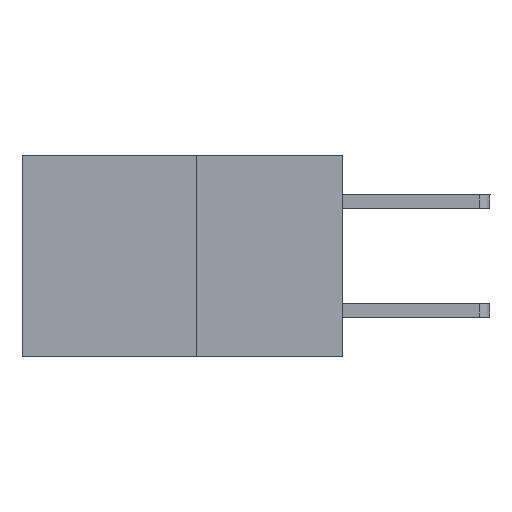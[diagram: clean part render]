
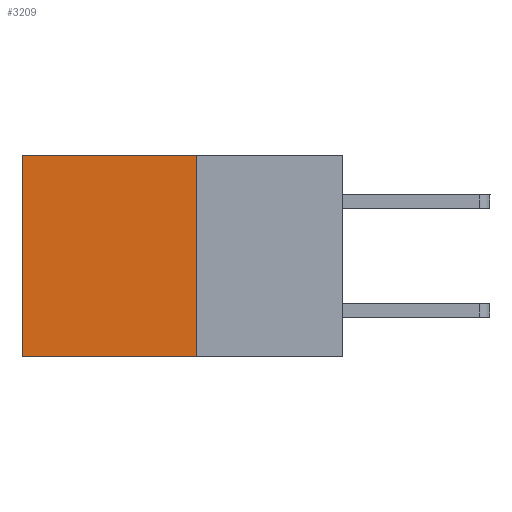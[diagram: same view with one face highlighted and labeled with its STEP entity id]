
A CAD part, left-side view. The second image highlights one B-rep face of the part: STEP entity #3209.
In plain terms, the highlighted planar face has unit normal (-1, 0, 0).
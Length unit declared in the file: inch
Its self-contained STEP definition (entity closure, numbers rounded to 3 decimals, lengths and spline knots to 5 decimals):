
#361 = VERTEX_POINT ( 'NONE', #5251 ) ;
#444 = CARTESIAN_POINT ( 'NONE',  ( 0.277, 0.27, -0.37 ) ) ;
#500 = DIRECTION ( 'NONE',  ( 0., 1., 0. ) ) ;
#676 = CARTESIAN_POINT ( 'NONE',  ( 0.277, 0.59, 0. ) ) ;
#831 = VERTEX_POINT ( 'NONE', #676 ) ;
#997 = VECTOR ( 'NONE', #500, 39.37008 ) ;
#1170 = ORIENTED_EDGE ( 'NONE', *, *, #3942, .F. ) ;
#1410 = LINE ( 'NONE', #3050, #6306 ) ;
#1750 = EDGE_CURVE ( 'NONE', #9320, #831, #1410, .T. ) ;
#1763 = LINE ( 'NONE', #9527, #6383 ) ;
#2321 = DIRECTION ( 'NONE',  ( 0., 0., -1. ) ) ;
#3050 = CARTESIAN_POINT ( 'NONE',  ( 0.277, 0.27, 0. ) ) ;
#3209 = ADVANCED_FACE ( 'NONE', ( #9004 ), #4160, .F. ) ;
#3211 = CARTESIAN_POINT ( 'NONE',  ( 0.277, 0.27, -0.37 ) ) ;
#3627 = ORIENTED_EDGE ( 'NONE', *, *, #1750, .T. ) ;
#3789 = DIRECTION ( 'NONE',  ( 0., 0., -1. ) ) ;
#3942 = EDGE_CURVE ( 'NONE', #9320, #361, #9128, .T. ) ;
#4008 = DIRECTION ( 'NONE',  ( 0., 0., -1. ) ) ;
#4160 = PLANE ( 'NONE',  #7378 ) ;
#4192 = CARTESIAN_POINT ( 'NONE',  ( 0.277, 0.27, -0.37 ) ) ;
#4925 = DIRECTION ( 'NONE',  ( 1., 0., 0. ) ) ;
#5251 = CARTESIAN_POINT ( 'NONE',  ( 0.277, 0.27, -0.37 ) ) ;
#5403 = CARTESIAN_POINT ( 'NONE',  ( 0.277, 0.59, -0.37 ) ) ;
#5517 = EDGE_LOOP ( 'NONE', ( #8155, #10459, #1170, #3627 ) ) ;
#6306 = VECTOR ( 'NONE', #8186, 39.37008 ) ;
#6383 = VECTOR ( 'NONE', #2321, 39.37008 ) ;
#6985 = EDGE_CURVE ( 'NONE', #361, #10839, #10267, .T. ) ;
#7378 = AXIS2_PLACEMENT_3D ( 'NONE', #4192, #4925, #4008 ) ;
#8155 = ORIENTED_EDGE ( 'NONE', *, *, #9687, .T. ) ;
#8186 = DIRECTION ( 'NONE',  ( 0., 1., 0. ) ) ;
#9004 = FACE_OUTER_BOUND ( 'NONE', #5517, .T. ) ;
#9128 = LINE ( 'NONE', #3211, #11412 ) ;
#9320 = VERTEX_POINT ( 'NONE', #10556 ) ;
#9527 = CARTESIAN_POINT ( 'NONE',  ( 0.277, 0.59, -0.37 ) ) ;
#9687 = EDGE_CURVE ( 'NONE', #831, #10839, #1763, .T. ) ;
#10267 = LINE ( 'NONE', #444, #997 ) ;
#10459 = ORIENTED_EDGE ( 'NONE', *, *, #6985, .F. ) ;
#10556 = CARTESIAN_POINT ( 'NONE',  ( 0.277, 0.27, 0. ) ) ;
#10839 = VERTEX_POINT ( 'NONE', #5403 ) ;
#11412 = VECTOR ( 'NONE', #3789, 39.37008 ) ;
